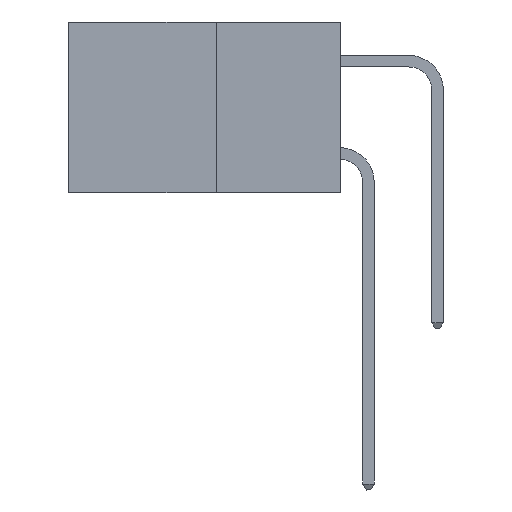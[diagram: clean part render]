
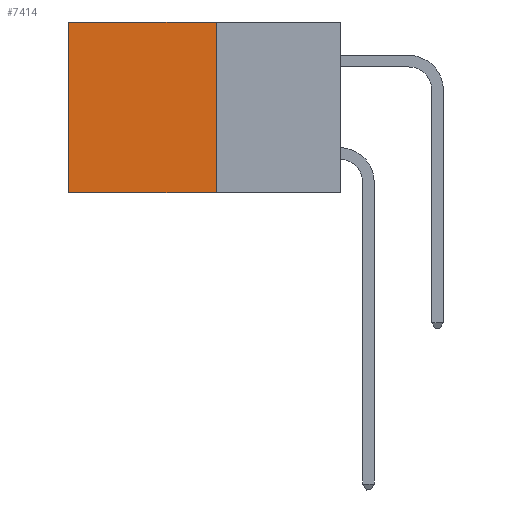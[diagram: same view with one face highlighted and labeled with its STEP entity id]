
A CAD part, left-side view. The second image highlights one B-rep face of the part: STEP entity #7414.
In plain terms, the highlighted planar face has unit normal (-1, 0, 0).
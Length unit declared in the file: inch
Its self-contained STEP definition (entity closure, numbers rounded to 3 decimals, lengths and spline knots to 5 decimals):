
#281 = CARTESIAN_POINT ( 'NONE',  ( 0.277, 0.59, -0.37 ) ) ;
#307 = LINE ( 'NONE', #12314, #9014 ) ;
#918 = VERTEX_POINT ( 'NONE', #13096 ) ;
#1196 = ORIENTED_EDGE ( 'NONE', *, *, #4317, .T. ) ;
#1479 = ORIENTED_EDGE ( 'NONE', *, *, #11629, .F. ) ;
#2758 = LINE ( 'NONE', #8855, #8236 ) ;
#3361 = CARTESIAN_POINT ( 'NONE',  ( 0.277, 0.27, -0.37 ) ) ;
#3363 = FACE_OUTER_BOUND ( 'NONE', #8738, .T. ) ;
#4317 = EDGE_CURVE ( 'NONE', #10458, #11062, #2758, .T. ) ;
#4808 = VERTEX_POINT ( 'NONE', #3361 ) ;
#4825 = CARTESIAN_POINT ( 'NONE',  ( 0.277, 0.27, -0.37 ) ) ;
#4974 = PLANE ( 'NONE',  #8676 ) ;
#5322 = DIRECTION ( 'NONE',  ( 0., 1., 0. ) ) ;
#5976 = DIRECTION ( 'NONE',  ( 0., 0., -1. ) ) ;
#6454 = LINE ( 'NONE', #10336, #12131 ) ;
#6767 = DIRECTION ( 'NONE',  ( 0., 0., -1. ) ) ;
#7414 = ADVANCED_FACE ( 'NONE', ( #3363 ), #4974, .F. ) ;
#7709 = EDGE_CURVE ( 'NONE', #4808, #918, #307, .T. ) ;
#8236 = VECTOR ( 'NONE', #5322, 39.37008 ) ;
#8354 = LINE ( 'NONE', #281, #13522 ) ;
#8676 = AXIS2_PLACEMENT_3D ( 'NONE', #4825, #10193, #12548 ) ;
#8738 = EDGE_LOOP ( 'NONE', ( #11765, #12184, #1479, #1196 ) ) ;
#8855 = CARTESIAN_POINT ( 'NONE',  ( 0.277, 0.27, 0. ) ) ;
#9014 = VECTOR ( 'NONE', #9706, 39.37008 ) ;
#9503 = CARTESIAN_POINT ( 'NONE',  ( 0.277, 0.27, 0. ) ) ;
#9706 = DIRECTION ( 'NONE',  ( 0., 1., 0. ) ) ;
#10193 = DIRECTION ( 'NONE',  ( 1., 0., 0. ) ) ;
#10336 = CARTESIAN_POINT ( 'NONE',  ( 0.277, 0.27, -0.37 ) ) ;
#10458 = VERTEX_POINT ( 'NONE', #9503 ) ;
#10537 = CARTESIAN_POINT ( 'NONE',  ( 0.277, 0.59, 0. ) ) ;
#11062 = VERTEX_POINT ( 'NONE', #10537 ) ;
#11629 = EDGE_CURVE ( 'NONE', #10458, #4808, #6454, .T. ) ;
#11765 = ORIENTED_EDGE ( 'NONE', *, *, #12076, .T. ) ;
#12076 = EDGE_CURVE ( 'NONE', #11062, #918, #8354, .T. ) ;
#12131 = VECTOR ( 'NONE', #5976, 39.37008 ) ;
#12184 = ORIENTED_EDGE ( 'NONE', *, *, #7709, .F. ) ;
#12314 = CARTESIAN_POINT ( 'NONE',  ( 0.277, 0.27, -0.37 ) ) ;
#12548 = DIRECTION ( 'NONE',  ( 0., 0., -1. ) ) ;
#13096 = CARTESIAN_POINT ( 'NONE',  ( 0.277, 0.59, -0.37 ) ) ;
#13522 = VECTOR ( 'NONE', #6767, 39.37008 ) ;
